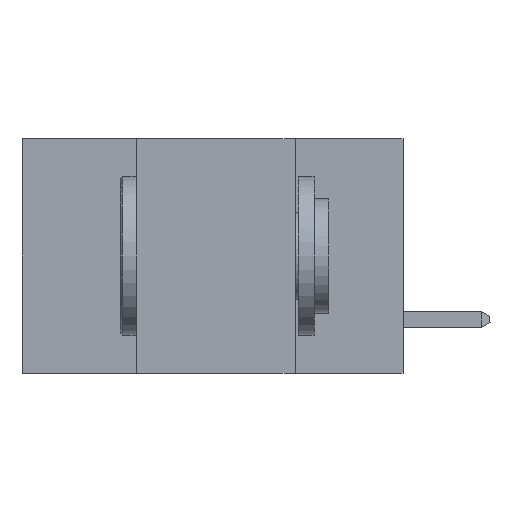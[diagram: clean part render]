
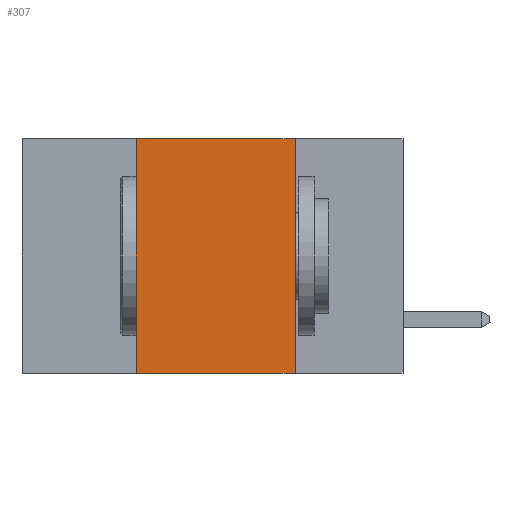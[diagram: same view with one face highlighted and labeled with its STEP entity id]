
A CAD part, left-side view. The second image highlights one B-rep face of the part: STEP entity #307.
In plain terms, the highlighted planar face has unit normal (-1, 0, 0).
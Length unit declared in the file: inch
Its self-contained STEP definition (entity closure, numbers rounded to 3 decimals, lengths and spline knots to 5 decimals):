
#1 = AXIS2_PLACEMENT_3D ( 'NONE', #8614, #1591, #3232 ) ;
#307 = ADVANCED_FACE ( 'NONE', ( #8397 ), #737, .F. ) ;
#382 = CARTESIAN_POINT ( 'NONE',  ( 0., 0.17, -0.37 ) ) ;
#737 = PLANE ( 'NONE',  #1 ) ;
#839 = VERTEX_POINT ( 'NONE', #1489 ) ;
#881 = VERTEX_POINT ( 'NONE', #4608 ) ;
#1489 = CARTESIAN_POINT ( 'NONE',  ( 0., 0.42, 0. ) ) ;
#1539 = ORIENTED_EDGE ( 'NONE', *, *, #3800, .F. ) ;
#1591 = DIRECTION ( 'NONE',  ( 1., 0., 0. ) ) ;
#1861 = DIRECTION ( 'NONE',  ( 0., 0., -1. ) ) ;
#2063 = EDGE_CURVE ( 'NONE', #839, #881, #4542, .T. ) ;
#2208 = EDGE_CURVE ( 'NONE', #5923, #7810, #5775, .T. ) ;
#2450 = VECTOR ( 'NONE', #9420, 39.37008 ) ;
#2807 = CARTESIAN_POINT ( 'NONE',  ( 0., 0.17, 0. ) ) ;
#3230 = CARTESIAN_POINT ( 'NONE',  ( 0., 0.6, -0.37 ) ) ;
#3232 = DIRECTION ( 'NONE',  ( 0., 0., -1. ) ) ;
#3800 = EDGE_CURVE ( 'NONE', #881, #7810, #5636, .T. ) ;
#4414 = VECTOR ( 'NONE', #8754, 39.37008 ) ;
#4539 = CARTESIAN_POINT ( 'NONE',  ( 0., 0.42, 0. ) ) ;
#4542 = LINE ( 'NONE', #9340, #2450 ) ;
#4608 = CARTESIAN_POINT ( 'NONE',  ( 0., 0.17, 0. ) ) ;
#5260 = EDGE_CURVE ( 'NONE', #5923, #839, #7955, .T. ) ;
#5567 = ORIENTED_EDGE ( 'NONE', *, *, #2208, .T. ) ;
#5636 = LINE ( 'NONE', #2807, #7983 ) ;
#5722 = CARTESIAN_POINT ( 'NONE',  ( 0., 0.42, -0.37 ) ) ;
#5775 = LINE ( 'NONE', #3230, #4414 ) ;
#5923 = VERTEX_POINT ( 'NONE', #5722 ) ;
#6307 = ORIENTED_EDGE ( 'NONE', *, *, #5260, .F. ) ;
#7205 = VECTOR ( 'NONE', #8685, 39.37008 ) ;
#7772 = ORIENTED_EDGE ( 'NONE', *, *, #2063, .F. ) ;
#7810 = VERTEX_POINT ( 'NONE', #382 ) ;
#7955 = LINE ( 'NONE', #4539, #7205 ) ;
#7983 = VECTOR ( 'NONE', #1861, 39.37008 ) ;
#8397 = FACE_OUTER_BOUND ( 'NONE', #10075, .T. ) ;
#8614 = CARTESIAN_POINT ( 'NONE',  ( 0., 0.6, 0. ) ) ;
#8685 = DIRECTION ( 'NONE',  ( 0., 0., 1. ) ) ;
#8754 = DIRECTION ( 'NONE',  ( 0., -1., 0. ) ) ;
#9340 = CARTESIAN_POINT ( 'NONE',  ( 0., 0.6, 0. ) ) ;
#9420 = DIRECTION ( 'NONE',  ( 0., -1., 0. ) ) ;
#10075 = EDGE_LOOP ( 'NONE', ( #1539, #7772, #6307, #5567 ) ) ;
